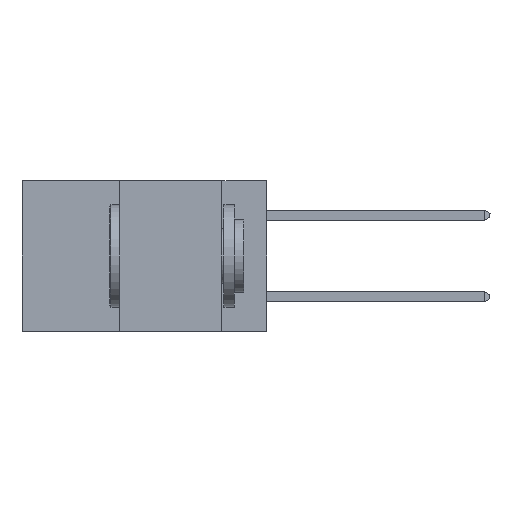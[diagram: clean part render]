
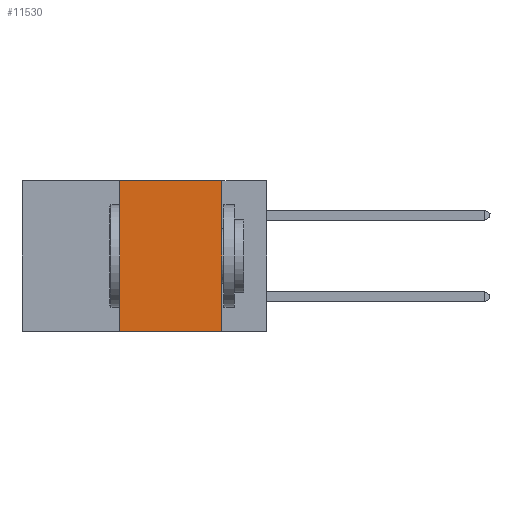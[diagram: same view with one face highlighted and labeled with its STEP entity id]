
A CAD part, left-side view. The second image highlights one B-rep face of the part: STEP entity #11530.
In plain terms, the highlighted planar face has unit normal (-1, 0, 0).
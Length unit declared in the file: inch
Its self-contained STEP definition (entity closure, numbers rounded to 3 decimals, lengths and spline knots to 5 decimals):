
#1249 = FACE_OUTER_BOUND ( 'NONE', #9620, .T. ) ;
#1530 = DIRECTION ( 'NONE',  ( 0., -1., 0. ) ) ;
#2298 = ORIENTED_EDGE ( 'NONE', *, *, #8770, .F. ) ;
#2479 = VERTEX_POINT ( 'NONE', #8034 ) ;
#3461 = VECTOR ( 'NONE', #8890, 39.37008 ) ;
#3554 = ORIENTED_EDGE ( 'NONE', *, *, #11497, .F. ) ;
#4501 = AXIS2_PLACEMENT_3D ( 'NONE', #10537, #5046, #12674 ) ;
#4774 = CARTESIAN_POINT ( 'NONE',  ( 0., 0.11, 0. ) ) ;
#5046 = DIRECTION ( 'NONE',  ( 1., 0., 0. ) ) ;
#5119 = VECTOR ( 'NONE', #8074, 39.37008 ) ;
#5551 = CARTESIAN_POINT ( 'NONE',  ( 0., 0.36, 0. ) ) ;
#6374 = ORIENTED_EDGE ( 'NONE', *, *, #10498, .F. ) ;
#7098 = EDGE_CURVE ( 'NONE', #8003, #2479, #9126, .T. ) ;
#7401 = CARTESIAN_POINT ( 'NONE',  ( 0., 0.6, -0.37 ) ) ;
#7648 = VECTOR ( 'NONE', #1530, 39.37008 ) ;
#7985 = LINE ( 'NONE', #8292, #7648 ) ;
#8003 = VERTEX_POINT ( 'NONE', #9005 ) ;
#8034 = CARTESIAN_POINT ( 'NONE',  ( 0., 0.11, -0.37 ) ) ;
#8066 = LINE ( 'NONE', #4774, #5119 ) ;
#8074 = DIRECTION ( 'NONE',  ( 0., 0., -1. ) ) ;
#8083 = VERTEX_POINT ( 'NONE', #11289 ) ;
#8292 = CARTESIAN_POINT ( 'NONE',  ( 0., 0.6, 0. ) ) ;
#8335 = PLANE ( 'NONE',  #4501 ) ;
#8475 = VERTEX_POINT ( 'NONE', #10856 ) ;
#8511 = DIRECTION ( 'NONE',  ( 0., -1., 0. ) ) ;
#8770 = EDGE_CURVE ( 'NONE', #8475, #2479, #8066, .T. ) ;
#8890 = DIRECTION ( 'NONE',  ( 0., 0., 1. ) ) ;
#9005 = CARTESIAN_POINT ( 'NONE',  ( 0., 0.36, -0.37 ) ) ;
#9126 = LINE ( 'NONE', #7401, #11679 ) ;
#9620 = EDGE_LOOP ( 'NONE', ( #2298, #3554, #6374, #11071 ) ) ;
#10498 = EDGE_CURVE ( 'NONE', #8003, #8083, #11257, .T. ) ;
#10537 = CARTESIAN_POINT ( 'NONE',  ( 0., 0.6, 0. ) ) ;
#10856 = CARTESIAN_POINT ( 'NONE',  ( 0., 0.11, 0. ) ) ;
#11071 = ORIENTED_EDGE ( 'NONE', *, *, #7098, .T. ) ;
#11257 = LINE ( 'NONE', #5551, #3461 ) ;
#11289 = CARTESIAN_POINT ( 'NONE',  ( 0., 0.36, 0. ) ) ;
#11497 = EDGE_CURVE ( 'NONE', #8083, #8475, #7985, .T. ) ;
#11530 = ADVANCED_FACE ( 'NONE', ( #1249 ), #8335, .F. ) ;
#11679 = VECTOR ( 'NONE', #8511, 39.37008 ) ;
#12674 = DIRECTION ( 'NONE',  ( 0., 0., -1. ) ) ;
